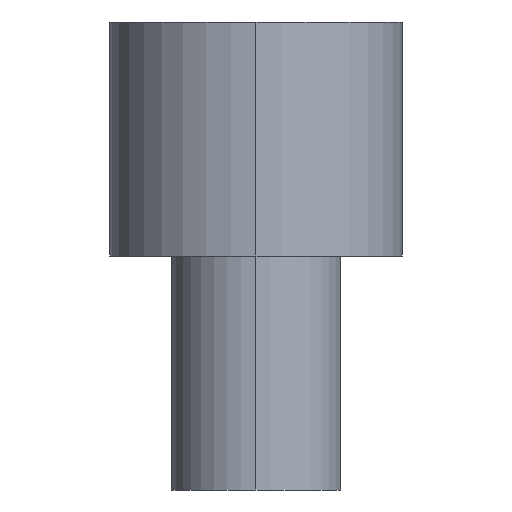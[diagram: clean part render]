
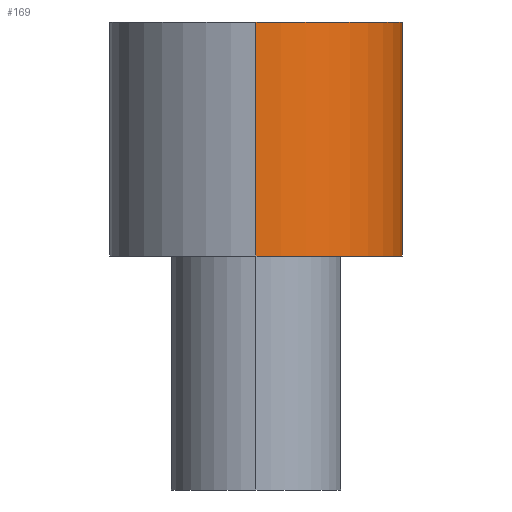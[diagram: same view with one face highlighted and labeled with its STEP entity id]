
A CAD part, left-side view. The second image highlights one B-rep face of the part: STEP entity #169.
In plain terms, the highlighted cylindrical face has radius 2.5 mm (diameter 5 mm), a partial arc.
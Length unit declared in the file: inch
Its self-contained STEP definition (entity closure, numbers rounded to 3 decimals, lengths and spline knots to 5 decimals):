
#3 = ORIENTED_EDGE ( 'NONE', *, *, #136, .T. ) ;
#11 = CIRCLE ( 'NONE', #321, 0.09843 ) ;
#13 = CARTESIAN_POINT ( 'NONE',  ( 0., 0., 0.31496 ) ) ;
#21 = DIRECTION ( 'NONE',  ( 0., 0., 1. ) ) ;
#23 = CARTESIAN_POINT ( 'NONE',  ( -0.09843, 0., 0.31496 ) ) ;
#29 = CIRCLE ( 'NONE', #31, 0.09843 ) ;
#31 = AXIS2_PLACEMENT_3D ( 'NONE', #13, #191, #40 ) ;
#32 = CARTESIAN_POINT ( 'NONE',  ( -0.09843, 0., 0.15748 ) ) ;
#40 = DIRECTION ( 'NONE',  ( 1., 0., 0. ) ) ;
#43 = EDGE_CURVE ( 'NONE', #213, #252, #29, .T. ) ;
#49 = EDGE_CURVE ( 'NONE', #252, #319, #189, .T. ) ;
#69 = CARTESIAN_POINT ( 'NONE',  ( 0., 0., 0.31496 ) ) ;
#74 = CARTESIAN_POINT ( 'NONE',  ( 0., -0.09843, 0.31496 ) ) ;
#79 = VECTOR ( 'NONE', #220, 39.37008 ) ;
#91 = EDGE_LOOP ( 'NONE', ( #224, #97, #3, #126 ) ) ;
#97 = ORIENTED_EDGE ( 'NONE', *, *, #118, .T. ) ;
#118 = EDGE_CURVE ( 'NONE', #213, #330, #215, .T. ) ;
#126 = ORIENTED_EDGE ( 'NONE', *, *, #49, .F. ) ;
#130 = CARTESIAN_POINT ( 'NONE',  ( 0., -0.09843, 0.15748 ) ) ;
#133 = FACE_OUTER_BOUND ( 'NONE', #91, .T. ) ;
#136 = EDGE_CURVE ( 'NONE', #330, #319, #11, .T. ) ;
#138 = VECTOR ( 'NONE', #283, 39.37008 ) ;
#140 = CARTESIAN_POINT ( 'NONE',  ( 0., -0.09843, 0.31496 ) ) ;
#169 = ADVANCED_FACE ( 'NONE', ( #133 ), #328, .T. ) ;
#173 = CARTESIAN_POINT ( 'NONE',  ( -0.09843, 0., 0.31496 ) ) ;
#176 = CARTESIAN_POINT ( 'NONE',  ( 0., 0., 0.15748 ) ) ;
#177 = DIRECTION ( 'NONE',  ( -1., 0., 0. ) ) ;
#189 = LINE ( 'NONE', #140, #138 ) ;
#191 = DIRECTION ( 'NONE',  ( 0., 0., 1. ) ) ;
#201 = DIRECTION ( 'NONE',  ( 1., 0., 0. ) ) ;
#213 = VERTEX_POINT ( 'NONE', #23 ) ;
#215 = LINE ( 'NONE', #173, #79 ) ;
#220 = DIRECTION ( 'NONE',  ( 0., 0., -1. ) ) ;
#224 = ORIENTED_EDGE ( 'NONE', *, *, #43, .F. ) ;
#252 = VERTEX_POINT ( 'NONE', #74 ) ;
#283 = DIRECTION ( 'NONE',  ( 0., 0., -1. ) ) ;
#309 = AXIS2_PLACEMENT_3D ( 'NONE', #69, #325, #177 ) ;
#319 = VERTEX_POINT ( 'NONE', #130 ) ;
#321 = AXIS2_PLACEMENT_3D ( 'NONE', #176, #21, #201 ) ;
#325 = DIRECTION ( 'NONE',  ( 0., 0., -1. ) ) ;
#328 = CYLINDRICAL_SURFACE ( 'NONE', #309, 0.09843 ) ;
#330 = VERTEX_POINT ( 'NONE', #32 ) ;
